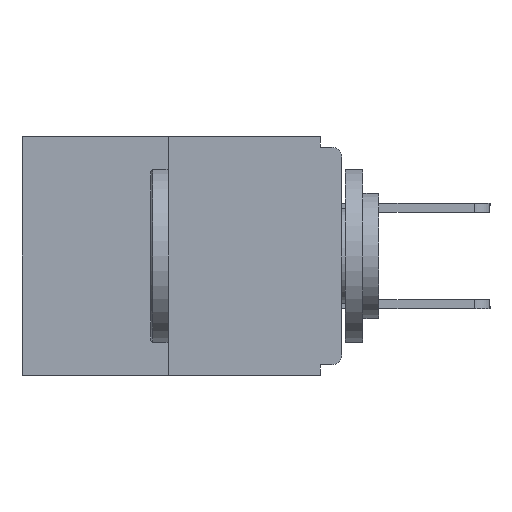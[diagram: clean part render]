
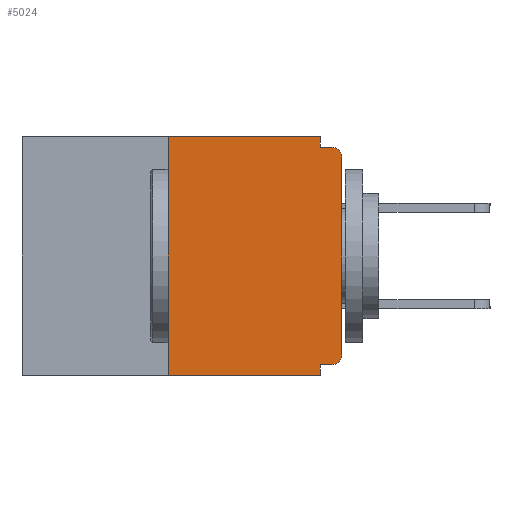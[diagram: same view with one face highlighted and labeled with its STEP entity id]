
A CAD part, left-side view. The second image highlights one B-rep face of the part: STEP entity #5024.
In plain terms, the highlighted planar face has unit normal (-1, 0, 0).
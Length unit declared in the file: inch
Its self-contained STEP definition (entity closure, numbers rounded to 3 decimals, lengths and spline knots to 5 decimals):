
#57 = FACE_OUTER_BOUND ( 'NONE', #5502, .T. ) ;
#111 = EDGE_CURVE ( 'NONE', #5782, #19419, #11253, .T. ) ;
#150 = EDGE_CURVE ( 'NONE', #7807, #2964, #11827, .T. ) ;
#330 = DIRECTION ( 'NONE',  ( 0., -1., 0. ) ) ;
#488 = CARTESIAN_POINT ( 'NONE',  ( 0., 0.031, -0.343 ) ) ;
#679 = CARTESIAN_POINT ( 'NONE',  ( 0., 0., -0.328 ) ) ;
#984 = CARTESIAN_POINT ( 'NONE',  ( 0., 0., -0.03 ) ) ;
#1068 = ORIENTED_EDGE ( 'NONE', *, *, #4265, .T. ) ;
#1742 = VECTOR ( 'NONE', #4021, 39.37008 ) ;
#2065 = CARTESIAN_POINT ( 'NONE',  ( 0., 0.46, 0. ) ) ;
#2659 = DIRECTION ( 'NONE',  ( 0., 0., -1. ) ) ;
#2908 = CARTESIAN_POINT ( 'NONE',  ( 0., 0.031, -0.343 ) ) ;
#2964 = VERTEX_POINT ( 'NONE', #5701 ) ;
#3108 = VECTOR ( 'NONE', #2659, 39.37008 ) ;
#3255 = VERTEX_POINT ( 'NONE', #2908 ) ;
#3507 = CARTESIAN_POINT ( 'NONE',  ( 0., 0.46, 0. ) ) ;
#4021 = DIRECTION ( 'NONE',  ( 0., -1., 0. ) ) ;
#4265 = EDGE_CURVE ( 'NONE', #8173, #5782, #8832, .T. ) ;
#4491 = DIRECTION ( 'NONE',  ( 0., 0., -1. ) ) ;
#4564 = CARTESIAN_POINT ( 'NONE',  ( 0., 0.031, -0.328 ) ) ;
#4734 = DIRECTION ( 'NONE',  ( -1., 0., 0. ) ) ;
#4856 = VECTOR ( 'NONE', #12806, 39.37008 ) ;
#4862 = ORIENTED_EDGE ( 'NONE', *, *, #6015, .F. ) ;
#5024 = ADVANCED_FACE ( 'NONE', ( #57 ), #12414, .F. ) ;
#5088 = DIRECTION ( 'NONE',  ( 1., 0., 0. ) ) ;
#5150 = EDGE_CURVE ( 'NONE', #13069, #9424, #9639, .T. ) ;
#5352 = VECTOR ( 'NONE', #12217, 39.37008 ) ;
#5502 = EDGE_LOOP ( 'NONE', ( #12972, #15482, #22820, #8046, #18972, #1068, #12463, #12273, #22929, #4862 ) ) ;
#5701 = CARTESIAN_POINT ( 'NONE',  ( 0., 0.25, 0. ) ) ;
#5782 = VERTEX_POINT ( 'NONE', #18158 ) ;
#5909 = DIRECTION ( 'NONE',  ( 0., 0., -1. ) ) ;
#6015 = EDGE_CURVE ( 'NONE', #21052, #13069, #14421, .T. ) ;
#6247 = LINE ( 'NONE', #14777, #7638 ) ;
#6312 = VERTEX_POINT ( 'NONE', #4564 ) ;
#6359 = CARTESIAN_POINT ( 'NONE',  ( 0., 0.015, -0.03 ) ) ;
#6537 = LINE ( 'NONE', #2065, #1742 ) ;
#6769 = AXIS2_PLACEMENT_3D ( 'NONE', #6359, #8319, #18983 ) ;
#7092 = VECTOR ( 'NONE', #5909, 39.37008 ) ;
#7638 = VECTOR ( 'NONE', #330, 39.37008 ) ;
#7731 = EDGE_CURVE ( 'NONE', #8173, #6312, #14081, .T. ) ;
#7807 = VERTEX_POINT ( 'NONE', #16856 ) ;
#8007 = CARTESIAN_POINT ( 'NONE',  ( 0., 0.031, 0. ) ) ;
#8046 = ORIENTED_EDGE ( 'NONE', *, *, #13960, .F. ) ;
#8173 = VERTEX_POINT ( 'NONE', #14209 ) ;
#8319 = DIRECTION ( 'NONE',  ( -1., 0., 0. ) ) ;
#8832 = CIRCLE ( 'NONE', #19036, 0.015 ) ;
#9424 = VERTEX_POINT ( 'NONE', #18055 ) ;
#9639 = LINE ( 'NONE', #23298, #4856 ) ;
#11253 = LINE ( 'NONE', #23024, #5352 ) ;
#11827 = LINE ( 'NONE', #17609, #19185 ) ;
#12217 = DIRECTION ( 'NONE',  ( 0., 0., 1. ) ) ;
#12273 = ORIENTED_EDGE ( 'NONE', *, *, #19413, .T. ) ;
#12414 = PLANE ( 'NONE',  #19343 ) ;
#12463 = ORIENTED_EDGE ( 'NONE', *, *, #111, .T. ) ;
#12806 = DIRECTION ( 'NONE',  ( 0., -1., 0. ) ) ;
#12972 = ORIENTED_EDGE ( 'NONE', *, *, #18711, .F. ) ;
#13069 = VERTEX_POINT ( 'NONE', #16894 ) ;
#13929 = EDGE_CURVE ( 'NONE', #7807, #3255, #6247, .T. ) ;
#13960 = EDGE_CURVE ( 'NONE', #6312, #3255, #18402, .T. ) ;
#14081 = LINE ( 'NONE', #679, #15781 ) ;
#14209 = CARTESIAN_POINT ( 'NONE',  ( 0., 0.015, -0.328 ) ) ;
#14421 = LINE ( 'NONE', #8007, #3108 ) ;
#14777 = CARTESIAN_POINT ( 'NONE',  ( 0., 0.46, -0.343 ) ) ;
#15482 = ORIENTED_EDGE ( 'NONE', *, *, #150, .F. ) ;
#15781 = VECTOR ( 'NONE', #22124, 39.37008 ) ;
#16856 = CARTESIAN_POINT ( 'NONE',  ( 0., 0.25, -0.343 ) ) ;
#16894 = CARTESIAN_POINT ( 'NONE',  ( 0., 0.031, -0.015 ) ) ;
#17609 = CARTESIAN_POINT ( 'NONE',  ( 0., 0.25, 0. ) ) ;
#18055 = CARTESIAN_POINT ( 'NONE',  ( 0., 0.015, -0.015 ) ) ;
#18158 = CARTESIAN_POINT ( 'NONE',  ( 0., 0., -0.313 ) ) ;
#18402 = LINE ( 'NONE', #488, #7092 ) ;
#18711 = EDGE_CURVE ( 'NONE', #2964, #21052, #6537, .T. ) ;
#18972 = ORIENTED_EDGE ( 'NONE', *, *, #7731, .F. ) ;
#18983 = DIRECTION ( 'NONE',  ( 0., 0., -1. ) ) ;
#19036 = AXIS2_PLACEMENT_3D ( 'NONE', #22636, #4734, #4491 ) ;
#19185 = VECTOR ( 'NONE', #19260, 39.37008 ) ;
#19260 = DIRECTION ( 'NONE',  ( 0., 0., 1. ) ) ;
#19343 = AXIS2_PLACEMENT_3D ( 'NONE', #3507, #5088, #19609 ) ;
#19413 = EDGE_CURVE ( 'NONE', #19419, #9424, #22053, .T. ) ;
#19419 = VERTEX_POINT ( 'NONE', #984 ) ;
#19609 = DIRECTION ( 'NONE',  ( 0., 0., -1. ) ) ;
#21052 = VERTEX_POINT ( 'NONE', #22898 ) ;
#22053 = CIRCLE ( 'NONE', #6769, 0.015 ) ;
#22124 = DIRECTION ( 'NONE',  ( 0., 1., 0. ) ) ;
#22636 = CARTESIAN_POINT ( 'NONE',  ( 0., 0.015, -0.313 ) ) ;
#22820 = ORIENTED_EDGE ( 'NONE', *, *, #13929, .T. ) ;
#22898 = CARTESIAN_POINT ( 'NONE',  ( 0., 0.031, 0. ) ) ;
#22929 = ORIENTED_EDGE ( 'NONE', *, *, #5150, .F. ) ;
#23024 = CARTESIAN_POINT ( 'NONE',  ( 0., 0., 0. ) ) ;
#23298 = CARTESIAN_POINT ( 'NONE',  ( 0., 0., -0.015 ) ) ;
